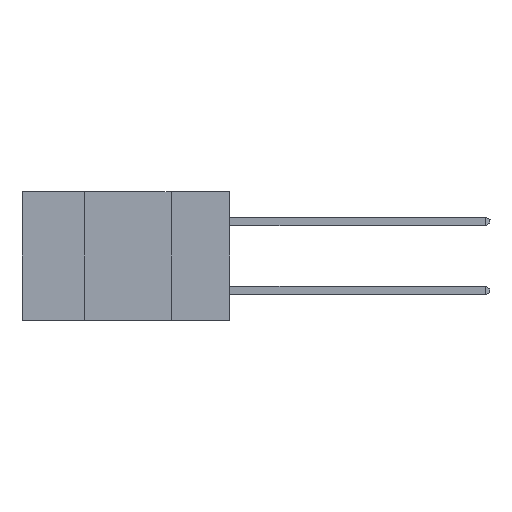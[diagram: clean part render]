
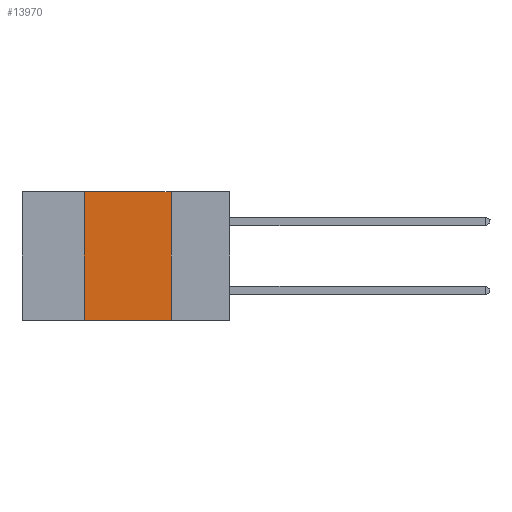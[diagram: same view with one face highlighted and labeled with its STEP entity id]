
A CAD part, left-side view. The second image highlights one B-rep face of the part: STEP entity #13970.
In plain terms, the highlighted planar face has unit normal (-1, 0, 0).
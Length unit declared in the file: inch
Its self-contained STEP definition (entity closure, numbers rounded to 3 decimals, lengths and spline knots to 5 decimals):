
#1272 = VECTOR ( 'NONE', #4584, 39.37008 ) ;
#2032 = CARTESIAN_POINT ( 'NONE',  ( 0., 0.42, 0. ) ) ;
#3600 = ORIENTED_EDGE ( 'NONE', *, *, #18271, .T. ) ;
#3604 = LINE ( 'NONE', #2032, #15662 ) ;
#4584 = DIRECTION ( 'NONE',  ( 0., -1., 0. ) ) ;
#5539 = VERTEX_POINT ( 'NONE', #22678 ) ;
#6129 = CARTESIAN_POINT ( 'NONE',  ( 0., 0.17, 0. ) ) ;
#6591 = VECTOR ( 'NONE', #20599, 39.37008 ) ;
#8061 = DIRECTION ( 'NONE',  ( 1., 0., 0. ) ) ;
#8479 = VECTOR ( 'NONE', #10147, 39.37008 ) ;
#9039 = AXIS2_PLACEMENT_3D ( 'NONE', #22559, #8061, #24970 ) ;
#9116 = CARTESIAN_POINT ( 'NONE',  ( 0., 0.17, -0.37 ) ) ;
#9120 = EDGE_CURVE ( 'NONE', #25763, #27642, #14939, .T. ) ;
#9538 = EDGE_CURVE ( 'NONE', #5539, #22918, #3604, .T. ) ;
#10147 = DIRECTION ( 'NONE',  ( 0., 0., -1. ) ) ;
#10901 = FACE_OUTER_BOUND ( 'NONE', #13134, .T. ) ;
#13134 = EDGE_LOOP ( 'NONE', ( #24707, #13364, #25126, #3600 ) ) ;
#13364 = ORIENTED_EDGE ( 'NONE', *, *, #22618, .F. ) ;
#13970 = ADVANCED_FACE ( 'NONE', ( #10901 ), #15263, .F. ) ;
#14060 = LINE ( 'NONE', #19021, #1272 ) ;
#14939 = LINE ( 'NONE', #19866, #8479 ) ;
#15263 = PLANE ( 'NONE',  #9039 ) ;
#15662 = VECTOR ( 'NONE', #21325, 39.37008 ) ;
#16874 = CARTESIAN_POINT ( 'NONE',  ( 0., 0.42, 0. ) ) ;
#18271 = EDGE_CURVE ( 'NONE', #5539, #27642, #14060, .T. ) ;
#18674 = LINE ( 'NONE', #25445, #6591 ) ;
#19021 = CARTESIAN_POINT ( 'NONE',  ( 0., 0.6, -0.37 ) ) ;
#19866 = CARTESIAN_POINT ( 'NONE',  ( 0., 0.17, 0. ) ) ;
#20599 = DIRECTION ( 'NONE',  ( 0., -1., 0. ) ) ;
#21325 = DIRECTION ( 'NONE',  ( 0., 0., 1. ) ) ;
#22559 = CARTESIAN_POINT ( 'NONE',  ( 0., 0.6, 0. ) ) ;
#22618 = EDGE_CURVE ( 'NONE', #22918, #25763, #18674, .T. ) ;
#22678 = CARTESIAN_POINT ( 'NONE',  ( 0., 0.42, -0.37 ) ) ;
#22918 = VERTEX_POINT ( 'NONE', #16874 ) ;
#24707 = ORIENTED_EDGE ( 'NONE', *, *, #9120, .F. ) ;
#24970 = DIRECTION ( 'NONE',  ( 0., 0., -1. ) ) ;
#25126 = ORIENTED_EDGE ( 'NONE', *, *, #9538, .F. ) ;
#25445 = CARTESIAN_POINT ( 'NONE',  ( 0., 0.6, 0. ) ) ;
#25763 = VERTEX_POINT ( 'NONE', #6129 ) ;
#27642 = VERTEX_POINT ( 'NONE', #9116 ) ;
